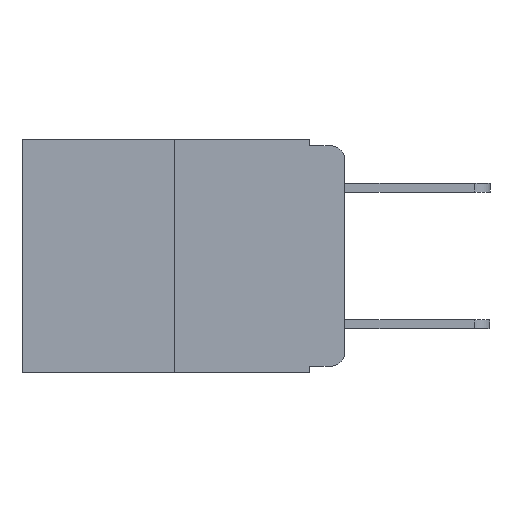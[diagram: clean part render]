
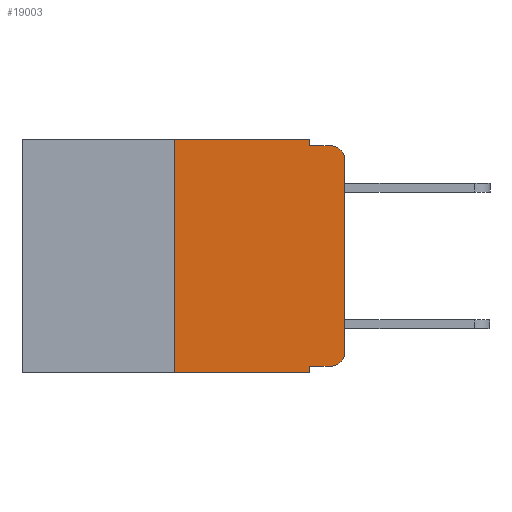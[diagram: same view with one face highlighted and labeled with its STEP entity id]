
A CAD part, left-side view. The second image highlights one B-rep face of the part: STEP entity #19003.
In plain terms, the highlighted planar face has unit normal (-1, 0, 0).
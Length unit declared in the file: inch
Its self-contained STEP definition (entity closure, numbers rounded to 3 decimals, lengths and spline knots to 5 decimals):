
#269 = VECTOR ( 'NONE', #13137, 39.37008 ) ;
#349 = DIRECTION ( 'NONE',  ( 0., -1., 0. ) ) ;
#1729 = VECTOR ( 'NONE', #13079, 39.37008 ) ;
#2318 = VERTEX_POINT ( 'NONE', #14350 ) ;
#2574 = CIRCLE ( 'NONE', #9156, 0.02 ) ;
#2575 = VERTEX_POINT ( 'NONE', #6116 ) ;
#2736 = DIRECTION ( 'NONE',  ( 0., 0., -1. ) ) ;
#2889 = VERTEX_POINT ( 'NONE', #19319 ) ;
#2937 = EDGE_CURVE ( 'NONE', #9663, #2889, #20155, .T. ) ;
#3164 = VERTEX_POINT ( 'NONE', #7818 ) ;
#4096 = ORIENTED_EDGE ( 'NONE', *, *, #5730, .F. ) ;
#4264 = CARTESIAN_POINT ( 'NONE',  ( 0., 0.473, 0. ) ) ;
#4437 = ORIENTED_EDGE ( 'NONE', *, *, #14489, .F. ) ;
#4492 = VERTEX_POINT ( 'NONE', #20409 ) ;
#4525 = CARTESIAN_POINT ( 'NONE',  ( 0., 0.051, -0.333 ) ) ;
#5021 = ORIENTED_EDGE ( 'NONE', *, *, #21916, .F. ) ;
#5036 = DIRECTION ( 'NONE',  ( -1., 0., 0. ) ) ;
#5680 = CARTESIAN_POINT ( 'NONE',  ( 0., 0.051, -0.333 ) ) ;
#5730 = EDGE_CURVE ( 'NONE', #19297, #9663, #11028, .T. ) ;
#5850 = VERTEX_POINT ( 'NONE', #13892 ) ;
#6116 = CARTESIAN_POINT ( 'NONE',  ( 0., 0.25, -0.343 ) ) ;
#6351 = LINE ( 'NONE', #5680, #14655 ) ;
#6769 = VECTOR ( 'NONE', #21951, 39.37008 ) ;
#6975 = ORIENTED_EDGE ( 'NONE', *, *, #18437, .T. ) ;
#7152 = ORIENTED_EDGE ( 'NONE', *, *, #18686, .F. ) ;
#7501 = CARTESIAN_POINT ( 'NONE',  ( 0., 0.051, -0.01 ) ) ;
#7741 = AXIS2_PLACEMENT_3D ( 'NONE', #19725, #9263, #21491 ) ;
#7818 = CARTESIAN_POINT ( 'NONE',  ( 0., 0.02, -0.333 ) ) ;
#8087 = CARTESIAN_POINT ( 'NONE',  ( 0., 0.051, 0. ) ) ;
#8180 = DIRECTION ( 'NONE',  ( 0., 0., -1. ) ) ;
#9005 = DIRECTION ( 'NONE',  ( 0., -1., 0. ) ) ;
#9156 = AXIS2_PLACEMENT_3D ( 'NONE', #15602, #5036, #17365 ) ;
#9263 = DIRECTION ( 'NONE',  ( -1., 0., 0. ) ) ;
#9532 = EDGE_LOOP ( 'NONE', ( #20094, #6975, #18867, #4096, #7152, #4437, #19835, #5021, #16415, #10374 ) ) ;
#9663 = VERTEX_POINT ( 'NONE', #7501 ) ;
#9692 = LINE ( 'NONE', #11334, #269 ) ;
#9868 = VERTEX_POINT ( 'NONE', #20531 ) ;
#10163 = DIRECTION ( 'NONE',  ( 0., -1., 0. ) ) ;
#10187 = EDGE_CURVE ( 'NONE', #21910, #3164, #6351, .T. ) ;
#10374 = ORIENTED_EDGE ( 'NONE', *, *, #19825, .T. ) ;
#10475 = VECTOR ( 'NONE', #8180, 39.37008 ) ;
#11028 = LINE ( 'NONE', #22178, #10475 ) ;
#11334 = CARTESIAN_POINT ( 'NONE',  ( 0., 0.25, 0. ) ) ;
#11729 = VECTOR ( 'NONE', #10163, 39.37008 ) ;
#11939 = CARTESIAN_POINT ( 'NONE',  ( 0., 0.473, -0.343 ) ) ;
#11967 = VECTOR ( 'NONE', #2736, 39.37008 ) ;
#12203 = DIRECTION ( 'NONE',  ( 0., 0., -1. ) ) ;
#13079 = DIRECTION ( 'NONE',  ( 0., -1., 0. ) ) ;
#13137 = DIRECTION ( 'NONE',  ( 0., 0., 1. ) ) ;
#13145 = CIRCLE ( 'NONE', #7741, 0.02 ) ;
#13350 = FACE_OUTER_BOUND ( 'NONE', #9532, .T. ) ;
#13892 = CARTESIAN_POINT ( 'NONE',  ( 0., 0., -0.03 ) ) ;
#14350 = CARTESIAN_POINT ( 'NONE',  ( 0., 0.25, 0. ) ) ;
#14489 = EDGE_CURVE ( 'NONE', #2575, #2318, #9692, .T. ) ;
#14655 = VECTOR ( 'NONE', #349, 39.37008 ) ;
#14740 = CARTESIAN_POINT ( 'NONE',  ( 0., 0.051, 0. ) ) ;
#14960 = CARTESIAN_POINT ( 'NONE',  ( 0., 0., 0. ) ) ;
#15545 = VECTOR ( 'NONE', #9005, 39.37008 ) ;
#15602 = CARTESIAN_POINT ( 'NONE',  ( 0., 0.02, -0.03 ) ) ;
#15815 = LINE ( 'NONE', #4264, #1729 ) ;
#15983 = CARTESIAN_POINT ( 'NONE',  ( 0., 0.051, -0.01 ) ) ;
#16132 = LINE ( 'NONE', #14960, #6769 ) ;
#16415 = ORIENTED_EDGE ( 'NONE', *, *, #10187, .T. ) ;
#17365 = DIRECTION ( 'NONE',  ( 0., 0., -1. ) ) ;
#17592 = EDGE_CURVE ( 'NONE', #9868, #5850, #16132, .T. ) ;
#18437 = EDGE_CURVE ( 'NONE', #5850, #2889, #2574, .T. ) ;
#18467 = AXIS2_PLACEMENT_3D ( 'NONE', #20909, #22647, #12203 ) ;
#18686 = EDGE_CURVE ( 'NONE', #2318, #19297, #15815, .T. ) ;
#18867 = ORIENTED_EDGE ( 'NONE', *, *, #2937, .F. ) ;
#19003 = ADVANCED_FACE ( 'NONE', ( #13350 ), #19139, .F. ) ;
#19139 = PLANE ( 'NONE',  #18467 ) ;
#19297 = VERTEX_POINT ( 'NONE', #14740 ) ;
#19319 = CARTESIAN_POINT ( 'NONE',  ( 0., 0.02, -0.01 ) ) ;
#19725 = CARTESIAN_POINT ( 'NONE',  ( 0., 0.02, -0.313 ) ) ;
#19825 = EDGE_CURVE ( 'NONE', #3164, #9868, #13145, .T. ) ;
#19835 = ORIENTED_EDGE ( 'NONE', *, *, #20140, .T. ) ;
#20094 = ORIENTED_EDGE ( 'NONE', *, *, #17592, .T. ) ;
#20140 = EDGE_CURVE ( 'NONE', #2575, #4492, #21569, .T. ) ;
#20155 = LINE ( 'NONE', #15983, #15545 ) ;
#20409 = CARTESIAN_POINT ( 'NONE',  ( 0., 0.051, -0.343 ) ) ;
#20531 = CARTESIAN_POINT ( 'NONE',  ( 0., 0., -0.313 ) ) ;
#20909 = CARTESIAN_POINT ( 'NONE',  ( 0., 0.473, 0. ) ) ;
#21257 = LINE ( 'NONE', #8087, #11967 ) ;
#21491 = DIRECTION ( 'NONE',  ( 0., 0., -1. ) ) ;
#21569 = LINE ( 'NONE', #11939, #11729 ) ;
#21910 = VERTEX_POINT ( 'NONE', #4525 ) ;
#21916 = EDGE_CURVE ( 'NONE', #21910, #4492, #21257, .T. ) ;
#21951 = DIRECTION ( 'NONE',  ( 0., 0., 1. ) ) ;
#22178 = CARTESIAN_POINT ( 'NONE',  ( 0., 0.051, 0. ) ) ;
#22647 = DIRECTION ( 'NONE',  ( 1., 0., 0. ) ) ;
